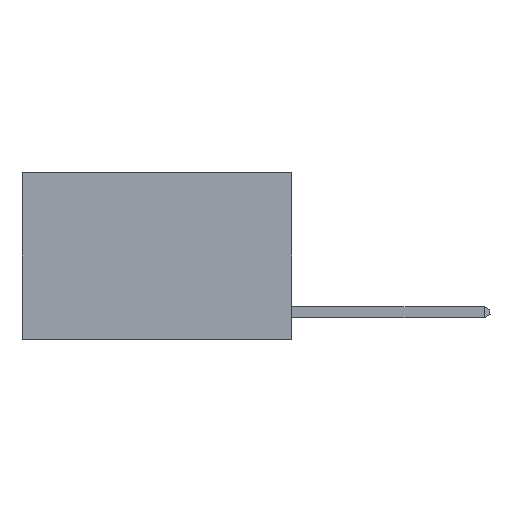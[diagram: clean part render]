
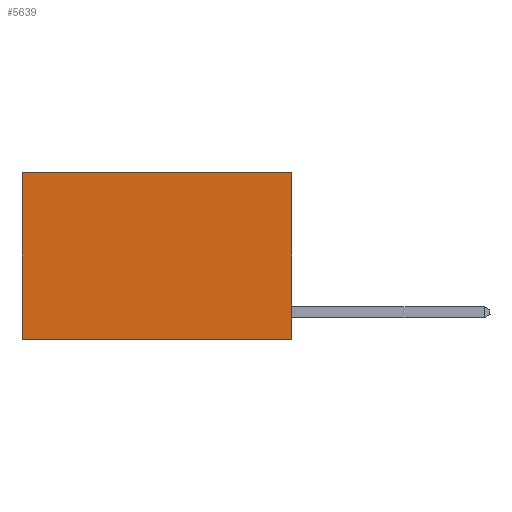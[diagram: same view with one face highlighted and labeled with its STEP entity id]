
A CAD part, left-side view. The second image highlights one B-rep face of the part: STEP entity #5639.
In plain terms, the highlighted planar face has unit normal (-1, 0, 0).
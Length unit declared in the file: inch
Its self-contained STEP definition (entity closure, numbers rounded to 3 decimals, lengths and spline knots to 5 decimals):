
#578 = VECTOR ( 'NONE', #8584, 39.37008 ) ;
#591 = ORIENTED_EDGE ( 'NONE', *, *, #8555, .F. ) ;
#1730 = ORIENTED_EDGE ( 'NONE', *, *, #12907, .T. ) ;
#2037 = VERTEX_POINT ( 'NONE', #15501 ) ;
#3527 = FACE_OUTER_BOUND ( 'NONE', #5356, .T. ) ;
#4106 = VECTOR ( 'NONE', #6551, 39.37008 ) ;
#5356 = EDGE_LOOP ( 'NONE', ( #12264, #12804, #591, #1730 ) ) ;
#5639 = ADVANCED_FACE ( 'NONE', ( #3527 ), #15583, .F. ) ;
#6072 = CARTESIAN_POINT ( 'NONE',  ( 0.2625, 0., 0. ) ) ;
#6321 = VECTOR ( 'NONE', #9649, 39.37008 ) ;
#6551 = DIRECTION ( 'NONE',  ( 0., 0., -1. ) ) ;
#7434 = DIRECTION ( 'NONE',  ( 1., 0., 0. ) ) ;
#7728 = LINE ( 'NONE', #11973, #4106 ) ;
#8170 = VERTEX_POINT ( 'NONE', #15947 ) ;
#8303 = LINE ( 'NONE', #10108, #11532 ) ;
#8398 = EDGE_CURVE ( 'NONE', #8170, #2037, #13548, .T. ) ;
#8555 = EDGE_CURVE ( 'NONE', #15321, #8170, #11440, .T. ) ;
#8584 = DIRECTION ( 'NONE',  ( 0., 0., -1. ) ) ;
#8740 = DIRECTION ( 'NONE',  ( 0., 1., 0. ) ) ;
#9453 = AXIS2_PLACEMENT_3D ( 'NONE', #6072, #7434, #16913 ) ;
#9592 = CARTESIAN_POINT ( 'NONE',  ( 0.2625, 0., -0.37 ) ) ;
#9649 = DIRECTION ( 'NONE',  ( 0., 1., 0. ) ) ;
#9946 = CARTESIAN_POINT ( 'NONE',  ( 0.2625, 0., 0. ) ) ;
#10108 = CARTESIAN_POINT ( 'NONE',  ( 0.2625, 0., 0. ) ) ;
#10297 = EDGE_CURVE ( 'NONE', #14194, #2037, #7728, .T. ) ;
#11337 = CARTESIAN_POINT ( 'NONE',  ( 0.2625, 0.6, 0. ) ) ;
#11440 = LINE ( 'NONE', #9946, #578 ) ;
#11532 = VECTOR ( 'NONE', #8740, 39.37008 ) ;
#11973 = CARTESIAN_POINT ( 'NONE',  ( 0.2625, 0.6, 0. ) ) ;
#12264 = ORIENTED_EDGE ( 'NONE', *, *, #10297, .T. ) ;
#12804 = ORIENTED_EDGE ( 'NONE', *, *, #8398, .F. ) ;
#12907 = EDGE_CURVE ( 'NONE', #15321, #14194, #8303, .T. ) ;
#13548 = LINE ( 'NONE', #9592, #6321 ) ;
#13716 = CARTESIAN_POINT ( 'NONE',  ( 0.2625, 0., 0. ) ) ;
#14194 = VERTEX_POINT ( 'NONE', #11337 ) ;
#15321 = VERTEX_POINT ( 'NONE', #13716 ) ;
#15501 = CARTESIAN_POINT ( 'NONE',  ( 0.2625, 0.6, -0.37 ) ) ;
#15583 = PLANE ( 'NONE',  #9453 ) ;
#15947 = CARTESIAN_POINT ( 'NONE',  ( 0.2625, 0., -0.37 ) ) ;
#16913 = DIRECTION ( 'NONE',  ( 0., 0., -1. ) ) ;
